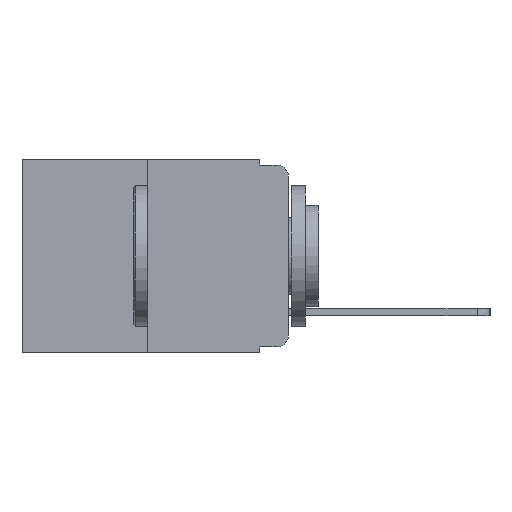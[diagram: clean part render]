
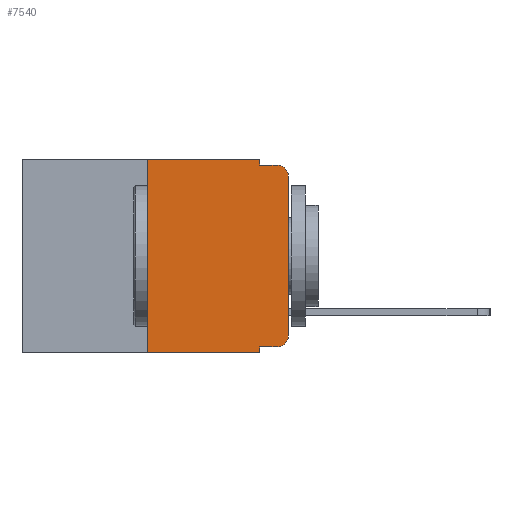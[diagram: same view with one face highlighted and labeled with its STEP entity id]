
A CAD part, left-side view. The second image highlights one B-rep face of the part: STEP entity #7540.
In plain terms, the highlighted planar face has unit normal (-1, 0, 0).
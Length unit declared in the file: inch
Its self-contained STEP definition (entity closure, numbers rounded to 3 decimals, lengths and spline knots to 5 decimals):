
#48 = LINE ( 'NONE', #8141, #3445 ) ;
#200 = LINE ( 'NONE', #18167, #4080 ) ;
#592 = VECTOR ( 'NONE', #13528, 39.37008 ) ;
#616 = DIRECTION ( 'NONE',  ( 0., -1., 0. ) ) ;
#1013 = DIRECTION ( 'NONE',  ( -1., 0., 0. ) ) ;
#1162 = CARTESIAN_POINT ( 'NONE',  ( 0., 0.473, -0.343 ) ) ;
#1554 = AXIS2_PLACEMENT_3D ( 'NONE', #9617, #1013, #11042 ) ;
#2175 = CIRCLE ( 'NONE', #5059, 0.02 ) ;
#2598 = VECTOR ( 'NONE', #9745, 39.37008 ) ;
#2759 = DIRECTION ( 'NONE',  ( 0., -1., 0. ) ) ;
#2916 = CARTESIAN_POINT ( 'NONE',  ( 0., 0.051, 0. ) ) ;
#3003 = CARTESIAN_POINT ( 'NONE',  ( 0., 0., 0. ) ) ;
#3209 = CARTESIAN_POINT ( 'NONE',  ( 0., 0.051, -0.333 ) ) ;
#3385 = EDGE_CURVE ( 'NONE', #14685, #12201, #4479, .T. ) ;
#3445 = VECTOR ( 'NONE', #9557, 39.37008 ) ;
#3554 = ORIENTED_EDGE ( 'NONE', *, *, #6517, .T. ) ;
#3634 = EDGE_CURVE ( 'NONE', #16768, #9047, #4236, .T. ) ;
#3750 = LINE ( 'NONE', #12066, #15104 ) ;
#4080 = VECTOR ( 'NONE', #11157, 39.37008 ) ;
#4126 = EDGE_CURVE ( 'NONE', #12136, #8663, #3750, .T. ) ;
#4236 = CIRCLE ( 'NONE', #1554, 0.02 ) ;
#4321 = LINE ( 'NONE', #17698, #15193 ) ;
#4428 = VERTEX_POINT ( 'NONE', #12803 ) ;
#4479 = LINE ( 'NONE', #10828, #592 ) ;
#4523 = DIRECTION ( 'NONE',  ( 0., 0., 1. ) ) ;
#5059 = AXIS2_PLACEMENT_3D ( 'NONE', #16376, #7921, #17813 ) ;
#5178 = ORIENTED_EDGE ( 'NONE', *, *, #10431, .F. ) ;
#5642 = EDGE_LOOP ( 'NONE', ( #9589, #15554, #14031, #12482, #7168, #5178, #7405, #9177, #3554, #13816 ) ) ;
#6517 = EDGE_CURVE ( 'NONE', #14685, #9564, #15232, .T. ) ;
#6805 = PLANE ( 'NONE',  #13201 ) ;
#7168 = ORIENTED_EDGE ( 'NONE', *, *, #7353, .F. ) ;
#7297 = CARTESIAN_POINT ( 'NONE',  ( 0., 0.051, -0.343 ) ) ;
#7353 = EDGE_CURVE ( 'NONE', #10113, #12136, #4321, .T. ) ;
#7405 = ORIENTED_EDGE ( 'NONE', *, *, #17142, .T. ) ;
#7540 = ADVANCED_FACE ( 'NONE', ( #9661 ), #6805, .F. ) ;
#7584 = EDGE_CURVE ( 'NONE', #8663, #9047, #200, .T. ) ;
#7921 = DIRECTION ( 'NONE',  ( -1., 0., 0. ) ) ;
#8141 = CARTESIAN_POINT ( 'NONE',  ( 0., 0.25, 0. ) ) ;
#8243 = DIRECTION ( 'NONE',  ( 0., 0., -1. ) ) ;
#8663 = VERTEX_POINT ( 'NONE', #10668 ) ;
#8898 = CARTESIAN_POINT ( 'NONE',  ( 0., 0., -0.03 ) ) ;
#9047 = VERTEX_POINT ( 'NONE', #10107 ) ;
#9177 = ORIENTED_EDGE ( 'NONE', *, *, #3385, .F. ) ;
#9557 = DIRECTION ( 'NONE',  ( 0., 0., 1. ) ) ;
#9564 = VERTEX_POINT ( 'NONE', #13109 ) ;
#9589 = ORIENTED_EDGE ( 'NONE', *, *, #17304, .T. ) ;
#9617 = CARTESIAN_POINT ( 'NONE',  ( 0., 0.02, -0.03 ) ) ;
#9661 = FACE_OUTER_BOUND ( 'NONE', #5642, .T. ) ;
#9745 = DIRECTION ( 'NONE',  ( 0., -1., 0. ) ) ;
#9885 = CARTESIAN_POINT ( 'NONE',  ( 0., 0.051, -0.333 ) ) ;
#10107 = CARTESIAN_POINT ( 'NONE',  ( 0., 0.02, -0.01 ) ) ;
#10113 = VERTEX_POINT ( 'NONE', #10244 ) ;
#10244 = CARTESIAN_POINT ( 'NONE',  ( 0., 0.25, 0. ) ) ;
#10400 = VECTOR ( 'NONE', #4523, 39.37008 ) ;
#10431 = EDGE_CURVE ( 'NONE', #12599, #10113, #48, .T. ) ;
#10668 = CARTESIAN_POINT ( 'NONE',  ( 0., 0.051, -0.01 ) ) ;
#10828 = CARTESIAN_POINT ( 'NONE',  ( 0., 0.051, 0. ) ) ;
#11028 = VECTOR ( 'NONE', #2759, 39.37008 ) ;
#11042 = DIRECTION ( 'NONE',  ( 0., 0., -1. ) ) ;
#11157 = DIRECTION ( 'NONE',  ( 0., -1., 0. ) ) ;
#12066 = CARTESIAN_POINT ( 'NONE',  ( 0., 0.051, 0. ) ) ;
#12136 = VERTEX_POINT ( 'NONE', #2916 ) ;
#12201 = VERTEX_POINT ( 'NONE', #7297 ) ;
#12482 = ORIENTED_EDGE ( 'NONE', *, *, #4126, .F. ) ;
#12599 = VERTEX_POINT ( 'NONE', #18145 ) ;
#12803 = CARTESIAN_POINT ( 'NONE',  ( 0., 0., -0.313 ) ) ;
#13109 = CARTESIAN_POINT ( 'NONE',  ( 0., 0.02, -0.333 ) ) ;
#13201 = AXIS2_PLACEMENT_3D ( 'NONE', #15292, #16696, #8243 ) ;
#13528 = DIRECTION ( 'NONE',  ( 0., 0., -1. ) ) ;
#13816 = ORIENTED_EDGE ( 'NONE', *, *, #16350, .T. ) ;
#14031 = ORIENTED_EDGE ( 'NONE', *, *, #7584, .F. ) ;
#14685 = VERTEX_POINT ( 'NONE', #3209 ) ;
#14853 = LINE ( 'NONE', #1162, #2598 ) ;
#15104 = VECTOR ( 'NONE', #17747, 39.37008 ) ;
#15193 = VECTOR ( 'NONE', #616, 39.37008 ) ;
#15232 = LINE ( 'NONE', #9885, #11028 ) ;
#15292 = CARTESIAN_POINT ( 'NONE',  ( 0., 0.473, 0. ) ) ;
#15554 = ORIENTED_EDGE ( 'NONE', *, *, #3634, .T. ) ;
#16350 = EDGE_CURVE ( 'NONE', #9564, #4428, #2175, .T. ) ;
#16376 = CARTESIAN_POINT ( 'NONE',  ( 0., 0.02, -0.313 ) ) ;
#16696 = DIRECTION ( 'NONE',  ( 1., 0., 0. ) ) ;
#16768 = VERTEX_POINT ( 'NONE', #8898 ) ;
#17142 = EDGE_CURVE ( 'NONE', #12599, #12201, #14853, .T. ) ;
#17304 = EDGE_CURVE ( 'NONE', #4428, #16768, #17924, .T. ) ;
#17698 = CARTESIAN_POINT ( 'NONE',  ( 0., 0.473, 0. ) ) ;
#17747 = DIRECTION ( 'NONE',  ( 0., 0., -1. ) ) ;
#17813 = DIRECTION ( 'NONE',  ( 0., 0., -1. ) ) ;
#17924 = LINE ( 'NONE', #3003, #10400 ) ;
#18145 = CARTESIAN_POINT ( 'NONE',  ( 0., 0.25, -0.343 ) ) ;
#18167 = CARTESIAN_POINT ( 'NONE',  ( 0., 0.051, -0.01 ) ) ;
